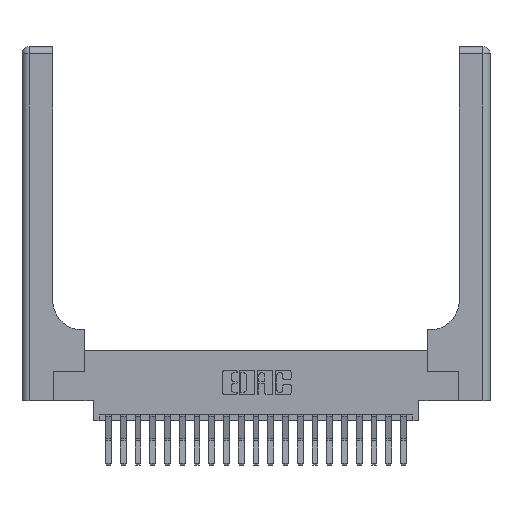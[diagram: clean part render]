
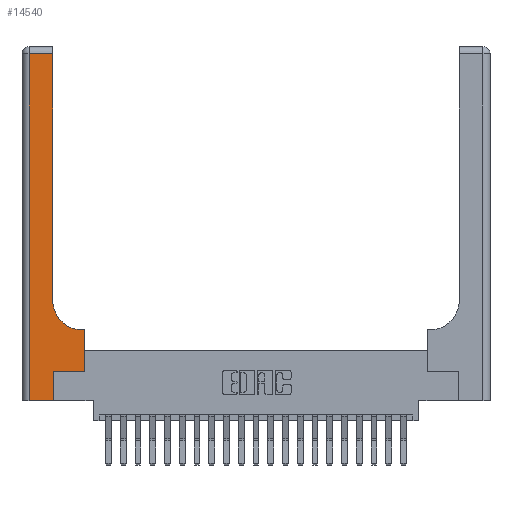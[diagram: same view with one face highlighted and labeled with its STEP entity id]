
A CAD part, top view. The second image highlights one B-rep face of the part: STEP entity #14540.
In plain terms, the highlighted planar face has unit normal (0, 0, 1).
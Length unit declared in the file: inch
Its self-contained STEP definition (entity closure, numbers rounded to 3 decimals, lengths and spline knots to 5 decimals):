
#229 = CARTESIAN_POINT ( 'NONE',  ( 0.26, 2.94, 0.37 ) ) ;
#548 = LINE ( 'NONE', #1042, #4565 ) ;
#653 = ORIENTED_EDGE ( 'NONE', *, *, #19969, .T. ) ;
#785 = VECTOR ( 'NONE', #16358, 39.37008 ) ;
#789 = AXIS2_PLACEMENT_3D ( 'NONE', #19766, #1113, #13019 ) ;
#1042 = CARTESIAN_POINT ( 'NONE',  ( 0.26, 0.6, 0.37 ) ) ;
#1113 = DIRECTION ( 'NONE',  ( 0., 0., -1. ) ) ;
#1206 = ORIENTED_EDGE ( 'NONE', *, *, #15155, .T. ) ;
#1272 = DIRECTION ( 'NONE',  ( 1., 0., 0. ) ) ;
#2197 = VECTOR ( 'NONE', #21547, 39.37008 ) ;
#2395 = LINE ( 'NONE', #7304, #11461 ) ;
#2554 = VERTEX_POINT ( 'NONE', #10005 ) ;
#2724 = CARTESIAN_POINT ( 'NONE',  ( 0.06, 2.94, 0.37 ) ) ;
#2822 = ORIENTED_EDGE ( 'NONE', *, *, #18956, .T. ) ;
#3050 = EDGE_CURVE ( 'NONE', #9729, #2554, #548, .T. ) ;
#3904 = CARTESIAN_POINT ( 'NONE',  ( 0.528, 0.25, 0.37 ) ) ;
#4445 = CARTESIAN_POINT ( 'NONE',  ( 0.265, 0., 0.37 ) ) ;
#4565 = VECTOR ( 'NONE', #19695, 39.37008 ) ;
#5024 = CARTESIAN_POINT ( 'NONE',  ( 0.528, 0.25, 0.37 ) ) ;
#5660 = CARTESIAN_POINT ( 'NONE',  ( 0.26, 3., 0.37 ) ) ;
#5667 = VERTEX_POINT ( 'NONE', #229 ) ;
#6534 = VERTEX_POINT ( 'NONE', #17960 ) ;
#6580 = EDGE_CURVE ( 'NONE', #5667, #8365, #17210, .T. ) ;
#7060 = ORIENTED_EDGE ( 'NONE', *, *, #11414, .T. ) ;
#7266 = LINE ( 'NONE', #16505, #2197 ) ;
#7304 = CARTESIAN_POINT ( 'NONE',  ( 0.06, 3., 0.37 ) ) ;
#7591 = ORIENTED_EDGE ( 'NONE', *, *, #6580, .T. ) ;
#7756 = FACE_OUTER_BOUND ( 'NONE', #13472, .T. ) ;
#7892 = ORIENTED_EDGE ( 'NONE', *, *, #3050, .T. ) ;
#7996 = CARTESIAN_POINT ( 'NONE',  ( 0.265, 0., 0.37 ) ) ;
#8365 = VERTEX_POINT ( 'NONE', #2724 ) ;
#8419 = ORIENTED_EDGE ( 'NONE', *, *, #20633, .T. ) ;
#8437 = DIRECTION ( 'NONE',  ( 1., 0., 0. ) ) ;
#8677 = ORIENTED_EDGE ( 'NONE', *, *, #8846, .T. ) ;
#8846 = EDGE_CURVE ( 'NONE', #8365, #19282, #2395, .T. ) ;
#9033 = DIRECTION ( 'NONE',  ( 0., -1., 0. ) ) ;
#9142 = VERTEX_POINT ( 'NONE', #7996 ) ;
#9729 = VERTEX_POINT ( 'NONE', #19830 ) ;
#10005 = CARTESIAN_POINT ( 'NONE',  ( 0.51, 0.6, 0.37 ) ) ;
#10714 = AXIS2_PLACEMENT_3D ( 'NONE', #21595, #11474, #1272 ) ;
#10715 = VERTEX_POINT ( 'NONE', #3904 ) ;
#11414 = EDGE_CURVE ( 'NONE', #14551, #5667, #15875, .T. ) ;
#11461 = VECTOR ( 'NONE', #9033, 39.37008 ) ;
#11474 = DIRECTION ( 'NONE',  ( 0., 0., -1. ) ) ;
#11501 = CIRCLE ( 'NONE', #10714, 0.25 ) ;
#11837 = VECTOR ( 'NONE', #15218, 39.37008 ) ;
#11838 = CARTESIAN_POINT ( 'NONE',  ( 0.265, 0.25, 0.37 ) ) ;
#13019 = DIRECTION ( 'NONE',  ( -1., 0., 0. ) ) ;
#13228 = VECTOR ( 'NONE', #14647, 39.37008 ) ;
#13325 = LINE ( 'NONE', #4445, #785 ) ;
#13472 = EDGE_LOOP ( 'NONE', ( #7060, #7591, #8677, #653, #1206, #19831, #2822, #7892, #8419 ) ) ;
#14540 = ADVANCED_FACE ( 'NONE', ( #7756 ), #21432, .F. ) ;
#14551 = VERTEX_POINT ( 'NONE', #14752 ) ;
#14647 = DIRECTION ( 'NONE',  ( -1., 0., 0. ) ) ;
#14752 = CARTESIAN_POINT ( 'NONE',  ( 0.26, 0.85, 0.37 ) ) ;
#15155 = EDGE_CURVE ( 'NONE', #9142, #6534, #13325, .T. ) ;
#15218 = DIRECTION ( 'NONE',  ( 0., 1., 0. ) ) ;
#15859 = DIRECTION ( 'NONE',  ( 0., 1., 0. ) ) ;
#15875 = LINE ( 'NONE', #5660, #18789 ) ;
#16358 = DIRECTION ( 'NONE',  ( 0., 1., 0. ) ) ;
#16385 = LINE ( 'NONE', #5024, #11837 ) ;
#16505 = CARTESIAN_POINT ( 'NONE',  ( 0., 0., 0.37 ) ) ;
#17023 = EDGE_CURVE ( 'NONE', #6534, #10715, #18044, .T. ) ;
#17210 = LINE ( 'NONE', #19728, #13228 ) ;
#17260 = CARTESIAN_POINT ( 'NONE',  ( 0.06, 0., 0.37 ) ) ;
#17960 = CARTESIAN_POINT ( 'NONE',  ( 0.265, 0.25, 0.37 ) ) ;
#18044 = LINE ( 'NONE', #11838, #21960 ) ;
#18789 = VECTOR ( 'NONE', #15859, 39.37008 ) ;
#18956 = EDGE_CURVE ( 'NONE', #10715, #9729, #16385, .T. ) ;
#19282 = VERTEX_POINT ( 'NONE', #17260 ) ;
#19695 = DIRECTION ( 'NONE',  ( -1., 0., 0. ) ) ;
#19728 = CARTESIAN_POINT ( 'NONE',  ( 0., 2.94, 0.37 ) ) ;
#19766 = CARTESIAN_POINT ( 'NONE',  ( 0., 3., 0.37 ) ) ;
#19830 = CARTESIAN_POINT ( 'NONE',  ( 0.528, 0.6, 0.37 ) ) ;
#19831 = ORIENTED_EDGE ( 'NONE', *, *, #17023, .T. ) ;
#19969 = EDGE_CURVE ( 'NONE', #19282, #9142, #7266, .T. ) ;
#20633 = EDGE_CURVE ( 'NONE', #2554, #14551, #11501, .T. ) ;
#21432 = PLANE ( 'NONE',  #789 ) ;
#21547 = DIRECTION ( 'NONE',  ( 1., 0., 0. ) ) ;
#21595 = CARTESIAN_POINT ( 'NONE',  ( 0.51, 0.85, 0.37 ) ) ;
#21960 = VECTOR ( 'NONE', #8437, 39.37008 ) ;
